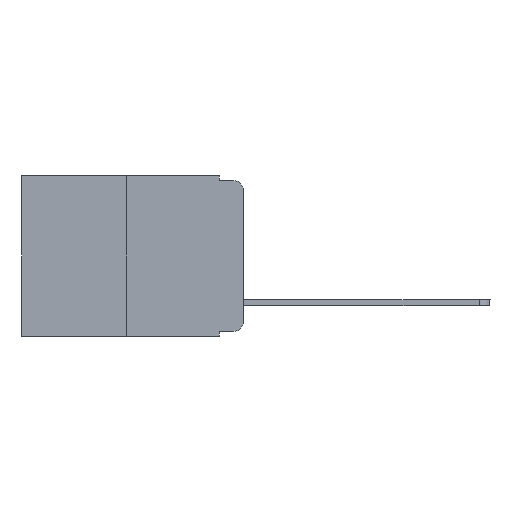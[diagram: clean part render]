
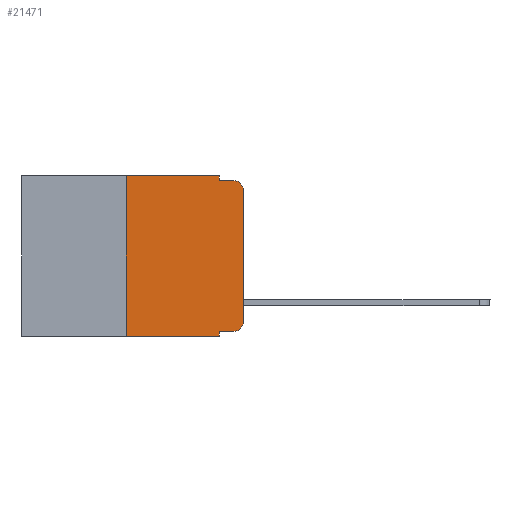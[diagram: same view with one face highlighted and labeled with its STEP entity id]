
A CAD part, left-side view. The second image highlights one B-rep face of the part: STEP entity #21471.
In plain terms, the highlighted planar face has unit normal (-1, 0, 0).
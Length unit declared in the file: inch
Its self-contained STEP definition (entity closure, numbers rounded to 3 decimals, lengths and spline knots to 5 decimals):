
#357 = VERTEX_POINT ( 'NONE', #3153 ) ;
#524 = VECTOR ( 'NONE', #8471, 39.37008 ) ;
#1197 = DIRECTION ( 'NONE',  ( -1., 0., 0. ) ) ;
#1415 = EDGE_CURVE ( 'NONE', #9381, #8189, #21124, .T. ) ;
#1871 = ORIENTED_EDGE ( 'NONE', *, *, #20038, .T. ) ;
#2079 = CARTESIAN_POINT ( 'NONE',  ( 0., 0.051, -0.343 ) ) ;
#2280 = CARTESIAN_POINT ( 'NONE',  ( 0., 0.02, -0.313 ) ) ;
#2500 = LINE ( 'NONE', #10163, #17630 ) ;
#2929 = CARTESIAN_POINT ( 'NONE',  ( 0., 0.02, -0.333 ) ) ;
#3044 = VERTEX_POINT ( 'NONE', #8909 ) ;
#3056 = VECTOR ( 'NONE', #24538, 39.37008 ) ;
#3153 = CARTESIAN_POINT ( 'NONE',  ( 0., 0., -0.03 ) ) ;
#3189 = VERTEX_POINT ( 'NONE', #9783 ) ;
#3226 = LINE ( 'NONE', #20629, #17681 ) ;
#3688 = VERTEX_POINT ( 'NONE', #2079 ) ;
#4201 = ORIENTED_EDGE ( 'NONE', *, *, #11611, .T. ) ;
#4484 = CARTESIAN_POINT ( 'NONE',  ( 0., 0.051, -0.333 ) ) ;
#4631 = EDGE_CURVE ( 'NONE', #22751, #9381, #12065, .T. ) ;
#4842 = EDGE_LOOP ( 'NONE', ( #9736, #6332, #21811, #13870, #8916, #21249, #1871, #19610, #4201, #14414 ) ) ;
#5446 = EDGE_CURVE ( 'NONE', #13473, #3189, #19588, .T. ) ;
#5551 = LINE ( 'NONE', #24362, #12380 ) ;
#5592 = LINE ( 'NONE', #7732, #24224 ) ;
#5601 = CARTESIAN_POINT ( 'NONE',  ( 0., 0.473, 0. ) ) ;
#6058 = LINE ( 'NONE', #13498, #14317 ) ;
#6329 = CARTESIAN_POINT ( 'NONE',  ( 0., 0.051, -0.01 ) ) ;
#6332 = ORIENTED_EDGE ( 'NONE', *, *, #17772, .T. ) ;
#6389 = DIRECTION ( 'NONE',  ( 0., 0., 1. ) ) ;
#7320 = DIRECTION ( 'NONE',  ( 0., 0., 1. ) ) ;
#7732 = CARTESIAN_POINT ( 'NONE',  ( 0., 0.051, 0. ) ) ;
#8189 = VERTEX_POINT ( 'NONE', #19703 ) ;
#8191 = DIRECTION ( 'NONE',  ( 0., 0., -1. ) ) ;
#8471 = DIRECTION ( 'NONE',  ( 0., -1., 0. ) ) ;
#8909 = CARTESIAN_POINT ( 'NONE',  ( 0., 0., -0.313 ) ) ;
#8916 = ORIENTED_EDGE ( 'NONE', *, *, #1415, .F. ) ;
#9381 = VERTEX_POINT ( 'NONE', #23406 ) ;
#9736 = ORIENTED_EDGE ( 'NONE', *, *, #10745, .T. ) ;
#9783 = CARTESIAN_POINT ( 'NONE',  ( 0., 0.02, -0.01 ) ) ;
#10151 = CARTESIAN_POINT ( 'NONE',  ( 0., 0.25, 0. ) ) ;
#10163 = CARTESIAN_POINT ( 'NONE',  ( 0., 0.051, 0. ) ) ;
#10355 = AXIS2_PLACEMENT_3D ( 'NONE', #2280, #17671, #8191 ) ;
#10745 = EDGE_CURVE ( 'NONE', #3044, #357, #5551, .T. ) ;
#10896 = EDGE_CURVE ( 'NONE', #13780, #3044, #21677, .T. ) ;
#10937 = PLANE ( 'NONE',  #11978 ) ;
#11025 = DIRECTION ( 'NONE',  ( 0., -1., 0. ) ) ;
#11611 = EDGE_CURVE ( 'NONE', #17722, #13780, #3226, .T. ) ;
#11978 = AXIS2_PLACEMENT_3D ( 'NONE', #17146, #16636, #20933 ) ;
#12065 = LINE ( 'NONE', #10151, #15417 ) ;
#12190 = DIRECTION ( 'NONE',  ( 0., 0., -1. ) ) ;
#12380 = VECTOR ( 'NONE', #7320, 39.37008 ) ;
#13473 = VERTEX_POINT ( 'NONE', #19345 ) ;
#13498 = CARTESIAN_POINT ( 'NONE',  ( 0., 0.473, -0.343 ) ) ;
#13780 = VERTEX_POINT ( 'NONE', #2929 ) ;
#13870 = ORIENTED_EDGE ( 'NONE', *, *, #21755, .F. ) ;
#14317 = VECTOR ( 'NONE', #15527, 39.37008 ) ;
#14414 = ORIENTED_EDGE ( 'NONE', *, *, #10896, .T. ) ;
#14671 = AXIS2_PLACEMENT_3D ( 'NONE', #16964, #1197, #15064 ) ;
#14708 = EDGE_CURVE ( 'NONE', #17722, #3688, #5592, .T. ) ;
#14988 = FACE_OUTER_BOUND ( 'NONE', #4842, .T. ) ;
#15064 = DIRECTION ( 'NONE',  ( 0., 0., -1. ) ) ;
#15417 = VECTOR ( 'NONE', #6389, 39.37008 ) ;
#15527 = DIRECTION ( 'NONE',  ( 0., -1., 0. ) ) ;
#16636 = DIRECTION ( 'NONE',  ( 1., 0., 0. ) ) ;
#16964 = CARTESIAN_POINT ( 'NONE',  ( 0., 0.02, -0.03 ) ) ;
#17124 = CIRCLE ( 'NONE', #14671, 0.02 ) ;
#17146 = CARTESIAN_POINT ( 'NONE',  ( 0., 0.473, 0. ) ) ;
#17630 = VECTOR ( 'NONE', #12190, 39.37008 ) ;
#17671 = DIRECTION ( 'NONE',  ( -1., 0., 0. ) ) ;
#17681 = VECTOR ( 'NONE', #11025, 39.37008 ) ;
#17722 = VERTEX_POINT ( 'NONE', #4484 ) ;
#17772 = EDGE_CURVE ( 'NONE', #357, #3189, #17124, .T. ) ;
#19345 = CARTESIAN_POINT ( 'NONE',  ( 0., 0.051, -0.01 ) ) ;
#19588 = LINE ( 'NONE', #6329, #524 ) ;
#19610 = ORIENTED_EDGE ( 'NONE', *, *, #14708, .F. ) ;
#19703 = CARTESIAN_POINT ( 'NONE',  ( 0., 0.051, 0. ) ) ;
#20038 = EDGE_CURVE ( 'NONE', #22751, #3688, #6058, .T. ) ;
#20629 = CARTESIAN_POINT ( 'NONE',  ( 0., 0.051, -0.333 ) ) ;
#20933 = DIRECTION ( 'NONE',  ( 0., 0., -1. ) ) ;
#20992 = DIRECTION ( 'NONE',  ( 0., 0., -1. ) ) ;
#21124 = LINE ( 'NONE', #5601, #3056 ) ;
#21249 = ORIENTED_EDGE ( 'NONE', *, *, #4631, .F. ) ;
#21471 = ADVANCED_FACE ( 'NONE', ( #14988 ), #10937, .F. ) ;
#21677 = CIRCLE ( 'NONE', #10355, 0.02 ) ;
#21755 = EDGE_CURVE ( 'NONE', #8189, #13473, #2500, .T. ) ;
#21811 = ORIENTED_EDGE ( 'NONE', *, *, #5446, .F. ) ;
#22751 = VERTEX_POINT ( 'NONE', #23358 ) ;
#23358 = CARTESIAN_POINT ( 'NONE',  ( 0., 0.25, -0.343 ) ) ;
#23406 = CARTESIAN_POINT ( 'NONE',  ( 0., 0.25, 0. ) ) ;
#24224 = VECTOR ( 'NONE', #20992, 39.37008 ) ;
#24362 = CARTESIAN_POINT ( 'NONE',  ( 0., 0., 0. ) ) ;
#24538 = DIRECTION ( 'NONE',  ( 0., -1., 0. ) ) ;
